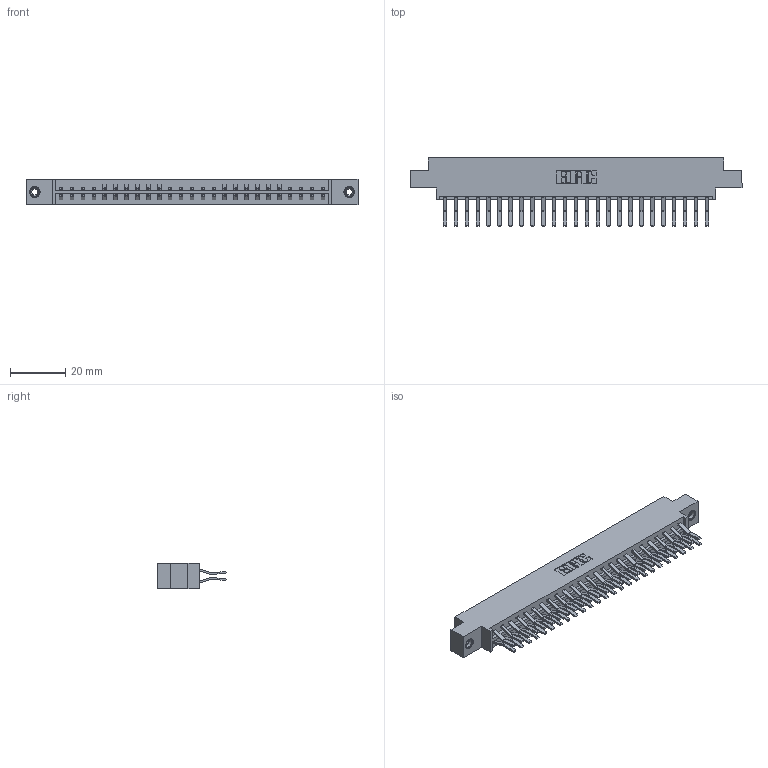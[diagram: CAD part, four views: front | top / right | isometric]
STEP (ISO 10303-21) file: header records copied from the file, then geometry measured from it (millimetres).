
FILE_DESCRIPTION (( 'STEP AP203' ), '1' );
FILE_NAME ('333-050-560-808.STEP', '2018-08-04T01:41:33', ( '' ), ( '' ), 'SwSTEP 2.0', 'SolidWorks 2016', '' );
FILE_SCHEMA (( 'CONFIG_CONTROL_DESIGN' ));
Length unit declared in the file: inch
Products named in the file (4): 333 Part_Offset - .156 Dia - TI; 345-292-001_560 Tail; 345-250-001_345-250-003-102; 333-050-560-808
Assembly tree (53 placements, depth 2):
  333-050-560-808
    333 Part_Offset - .156 Dia - TI
    345-292-001_560 Tail  x50
    345-250-001_345-250-003-102  x2
Bounding box: 120.6 x 24.78 x 9.4 mm (x, y, z)
Volume: 12246.9 mm3; surface area: 15473.7 mm2
Topology: 53 solids, 53 shells, 2878 faces, 8509 edges, 5598 vertices
Faces by surface type: plane 1906, cylinder 956, cone 12, torus 4
Entity records: 19688 total; most frequent: CARTESIAN_POINT 3269, ORIENTED_EDGE 3198, DIRECTION 2857, EDGE_CURVE 1599, VECTOR 1447, LINE 1447, VERTEX_POINT 1060, AXIS2_PLACEMENT_3D 705
